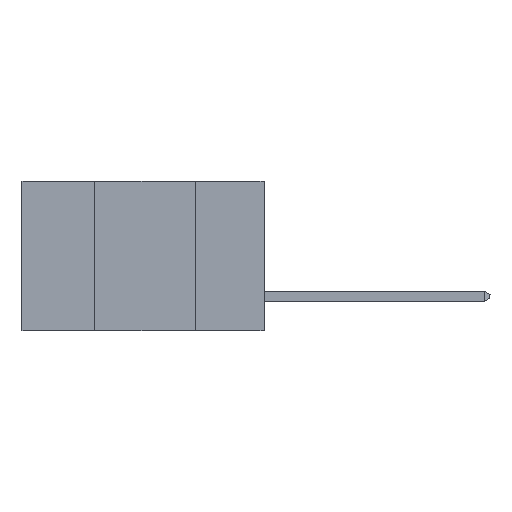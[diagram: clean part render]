
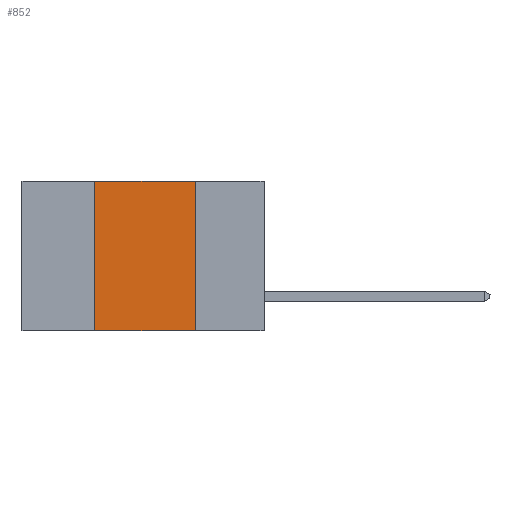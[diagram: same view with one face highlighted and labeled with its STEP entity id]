
A CAD part, left-side view. The second image highlights one B-rep face of the part: STEP entity #852.
In plain terms, the highlighted planar face has unit normal (-1, 0, 0).
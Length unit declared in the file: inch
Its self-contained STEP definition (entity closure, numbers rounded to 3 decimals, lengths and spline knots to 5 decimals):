
#183 = DIRECTION ( 'NONE',  ( 0., -1., 0. ) ) ;
#333 = CARTESIAN_POINT ( 'NONE',  ( 0., 0.17, 0. ) ) ;
#843 = CARTESIAN_POINT ( 'NONE',  ( 0., 0.17, -0.37 ) ) ;
#852 = ADVANCED_FACE ( 'NONE', ( #10977 ), #7618, .F. ) ;
#1372 = ORIENTED_EDGE ( 'NONE', *, *, #6997, .F. ) ;
#2083 = ORIENTED_EDGE ( 'NONE', *, *, #4422, .F. ) ;
#2308 = AXIS2_PLACEMENT_3D ( 'NONE', #6235, #11848, #11920 ) ;
#2343 = CARTESIAN_POINT ( 'NONE',  ( 0., 0.17, -0.37 ) ) ;
#2604 = VECTOR ( 'NONE', #10695, 39.37008 ) ;
#2685 = ORIENTED_EDGE ( 'NONE', *, *, #4005, .T. ) ;
#2740 = VERTEX_POINT ( 'NONE', #843 ) ;
#3641 = EDGE_CURVE ( 'NONE', #5527, #12107, #11740, .T. ) ;
#3680 = DIRECTION ( 'NONE',  ( 0., -1., 0. ) ) ;
#4005 = EDGE_CURVE ( 'NONE', #9079, #2740, #5549, .T. ) ;
#4150 = CARTESIAN_POINT ( 'NONE',  ( 0., 0.42, 0. ) ) ;
#4280 = ORIENTED_EDGE ( 'NONE', *, *, #3641, .F. ) ;
#4344 = DIRECTION ( 'NONE',  ( 0., 0., -1. ) ) ;
#4422 = EDGE_CURVE ( 'NONE', #9079, #5527, #7015, .T. ) ;
#5111 = EDGE_LOOP ( 'NONE', ( #1372, #4280, #2083, #2685 ) ) ;
#5399 = LINE ( 'NONE', #2343, #9398 ) ;
#5527 = VERTEX_POINT ( 'NONE', #4150 ) ;
#5549 = LINE ( 'NONE', #8418, #9797 ) ;
#6235 = CARTESIAN_POINT ( 'NONE',  ( 0., 0.6, 0. ) ) ;
#6997 = EDGE_CURVE ( 'NONE', #12107, #2740, #5399, .T. ) ;
#7015 = LINE ( 'NONE', #7951, #2604 ) ;
#7181 = CARTESIAN_POINT ( 'NONE',  ( 0., 0.42, -0.37 ) ) ;
#7618 = PLANE ( 'NONE',  #2308 ) ;
#7951 = CARTESIAN_POINT ( 'NONE',  ( 0., 0.42, -0.37 ) ) ;
#8418 = CARTESIAN_POINT ( 'NONE',  ( 0., 0.6, -0.37 ) ) ;
#9079 = VERTEX_POINT ( 'NONE', #7181 ) ;
#9398 = VECTOR ( 'NONE', #4344, 39.37008 ) ;
#9751 = CARTESIAN_POINT ( 'NONE',  ( 0., 0.6, 0. ) ) ;
#9797 = VECTOR ( 'NONE', #3680, 39.37008 ) ;
#9982 = VECTOR ( 'NONE', #183, 39.37008 ) ;
#10695 = DIRECTION ( 'NONE',  ( 0., 0., 1. ) ) ;
#10977 = FACE_OUTER_BOUND ( 'NONE', #5111, .T. ) ;
#11740 = LINE ( 'NONE', #9751, #9982 ) ;
#11848 = DIRECTION ( 'NONE',  ( 1., 0., 0. ) ) ;
#11920 = DIRECTION ( 'NONE',  ( 0., 0., -1. ) ) ;
#12107 = VERTEX_POINT ( 'NONE', #333 ) ;
